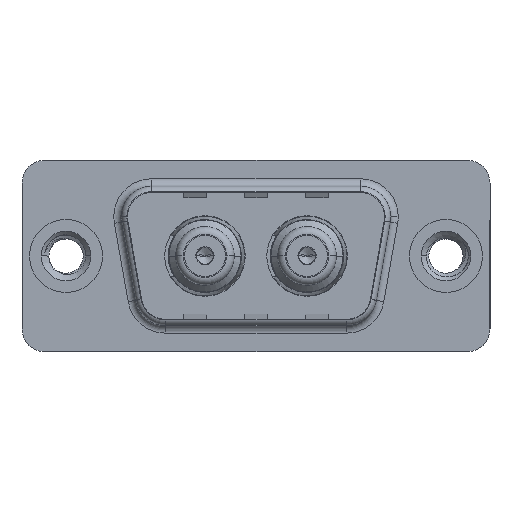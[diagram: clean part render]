
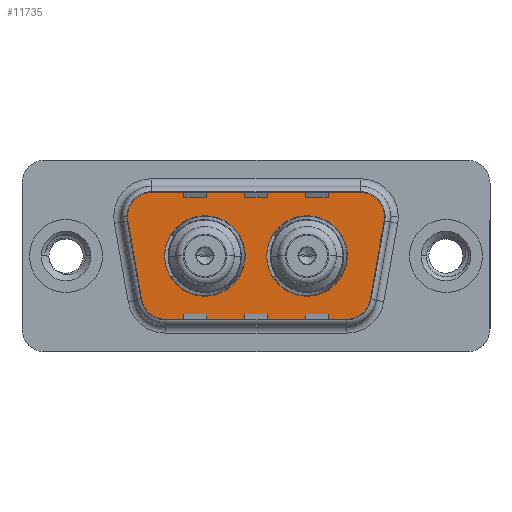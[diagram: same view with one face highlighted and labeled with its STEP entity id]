
A CAD part, top view. The second image highlights one B-rep face of the part: STEP entity #11735.
In plain terms, the highlighted planar face has unit normal (0, 0, 1).
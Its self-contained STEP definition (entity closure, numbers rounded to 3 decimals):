
#1 = CIRCLE ( 'NONE', #564, 2.65 ) ;
#114 = EDGE_CURVE ( 'NONE', #13973, #14673, #2329, .T. ) ;
#326 = VECTOR ( 'NONE', #3303, 1000. ) ;
#469 = DIRECTION ( 'NONE',  ( 0., 0., 1. ) ) ;
#486 = CARTESIAN_POINT ( 'NONE',  ( 19.564, 2.9, 0. ) ) ;
#564 = AXIS2_PLACEMENT_3D ( 'NONE', #6329, #6258, #6147 ) ;
#580 = FACE_BOUND ( 'NONE', #16173, .T. ) ;
#655 = DIRECTION ( 'NONE',  ( -1., 0., 0. ) ) ;
#695 = ORIENTED_EDGE ( 'NONE', *, *, #6274, .T. ) ;
#864 = CARTESIAN_POINT ( 'NONE',  ( 19.564, 2.9, 0. ) ) ;
#968 = CIRCLE ( 'NONE', #18307, 2. ) ;
#1324 = DIRECTION ( 'NONE',  ( 0., 0., 1. ) ) ;
#1358 = EDGE_CURVE ( 'NONE', #16031, #7079, #12045, .T. ) ;
#1480 = VERTEX_POINT ( 'NONE', #13743 ) ;
#1599 = ORIENTED_EDGE ( 'NONE', *, *, #8233, .F. ) ;
#1756 = CIRCLE ( 'NONE', #15174, 2. ) ;
#2310 = DIRECTION ( 'NONE',  ( -1., 0., 0. ) ) ;
#2329 = CIRCLE ( 'NONE', #5282, 2.65 ) ;
#2404 = CIRCLE ( 'NONE', #17236, 2.65 ) ;
#2619 = VERTEX_POINT ( 'NONE', #16301 ) ;
#2859 = CARTESIAN_POINT ( 'NONE',  ( 18.541, -2.9, 0. ) ) ;
#2981 = CARTESIAN_POINT ( 'NONE',  ( 5.436, 2.9, 0. ) ) ;
#3101 = CIRCLE ( 'NONE', #17448, 2. ) ;
#3128 = VECTOR ( 'NONE', #15255, 1000. ) ;
#3303 = DIRECTION ( 'NONE',  ( 0.174, -0.985, 0. ) ) ;
#3501 = FACE_BOUND ( 'NONE', #13004, .T. ) ;
#3754 = CARTESIAN_POINT ( 'NONE',  ( 5.436, 4.9, 0. ) ) ;
#4258 = DIRECTION ( 'NONE',  ( 1., 0., 0. ) ) ;
#4263 = EDGE_CURVE ( 'NONE', #13806, #17705, #1, .T. ) ;
#4389 = DIRECTION ( 'NONE',  ( 1., 0., 0. ) ) ;
#4454 = EDGE_CURVE ( 'NONE', #15812, #12667, #9995, .T. ) ;
#4488 = CIRCLE ( 'NONE', #15249, 2. ) ;
#4517 = CARTESIAN_POINT ( 'NONE',  ( 3.466, 2.553, 0. ) ) ;
#5018 = EDGE_CURVE ( 'NONE', #12593, #1480, #17698, .T. ) ;
#5043 = EDGE_CURVE ( 'NONE', #16084, #15812, #10149, .T. ) ;
#5282 = AXIS2_PLACEMENT_3D ( 'NONE', #17129, #10798, #13924 ) ;
#5322 = VECTOR ( 'NONE', #15487, 1000. ) ;
#5355 = CARTESIAN_POINT ( 'NONE',  ( 9.14, 0., 0. ) ) ;
#5369 = DIRECTION ( 'NONE',  ( -1., 0., 0. ) ) ;
#5607 = CARTESIAN_POINT ( 'NONE',  ( 21.534, 2.553, 0. ) ) ;
#5785 = VERTEX_POINT ( 'NONE', #6048 ) ;
#6048 = CARTESIAN_POINT ( 'NONE',  ( 21.534, 2.553, 0. ) ) ;
#6147 = DIRECTION ( 'NONE',  ( 1., 0., 0. ) ) ;
#6219 = ORIENTED_EDGE ( 'NONE', *, *, #18273, .T. ) ;
#6258 = DIRECTION ( 'NONE',  ( 0., 0., 1. ) ) ;
#6274 = EDGE_CURVE ( 'NONE', #1480, #2619, #3101, .T. ) ;
#6329 = CARTESIAN_POINT ( 'NONE',  ( 9.14, 0., 0. ) ) ;
#6382 = CARTESIAN_POINT ( 'NONE',  ( 6.459, -4.9, 0. ) ) ;
#6734 = DIRECTION ( 'NONE',  ( 1., 0., 0. ) ) ;
#7079 = VERTEX_POINT ( 'NONE', #10060 ) ;
#7116 = ORIENTED_EDGE ( 'NONE', *, *, #4454, .T. ) ;
#7161 = CARTESIAN_POINT ( 'NONE',  ( 18.51, 0., 0. ) ) ;
#7391 = CARTESIAN_POINT ( 'NONE',  ( 3.466, 2.553, 0. ) ) ;
#7783 = ORIENTED_EDGE ( 'NONE', *, *, #5043, .T. ) ;
#7798 = ORIENTED_EDGE ( 'NONE', *, *, #9588, .T. ) ;
#8108 = CARTESIAN_POINT ( 'NONE',  ( 6.459, -2.9, 0. ) ) ;
#8119 = CARTESIAN_POINT ( 'NONE',  ( 5.436, 4.9, 0. ) ) ;
#8124 = CARTESIAN_POINT ( 'NONE',  ( 15.86, 0., 0. ) ) ;
#8233 = EDGE_CURVE ( 'NONE', #14673, #13973, #2404, .T. ) ;
#8450 = ORIENTED_EDGE ( 'NONE', *, *, #16518, .T. ) ;
#8786 = CIRCLE ( 'NONE', #17103, 2.65 ) ;
#9030 = LINE ( 'NONE', #5607, #5322 ) ;
#9506 = DIRECTION ( 'NONE',  ( -1., 0., 0. ) ) ;
#9523 = DIRECTION ( 'NONE',  ( 1., 0., 0. ) ) ;
#9588 = EDGE_CURVE ( 'NONE', #7079, #12593, #1756, .T. ) ;
#9617 = EDGE_CURVE ( 'NONE', #17705, #13806, #8786, .T. ) ;
#9743 = CARTESIAN_POINT ( 'NONE',  ( 18.541, -2.9, 0. ) ) ;
#9995 = LINE ( 'NONE', #8119, #12392 ) ;
#10060 = CARTESIAN_POINT ( 'NONE',  ( 4.489, -3.247, 0. ) ) ;
#10149 = CIRCLE ( 'NONE', #12141, 2. ) ;
#10189 = ORIENTED_EDGE ( 'NONE', *, *, #4263, .F. ) ;
#10729 = DIRECTION ( 'NONE',  ( 0., 0., 1. ) ) ;
#10798 = DIRECTION ( 'NONE',  ( 0., 0., 1. ) ) ;
#11169 = DIRECTION ( 'NONE',  ( 1., 0., 0. ) ) ;
#11325 = CARTESIAN_POINT ( 'NONE',  ( 13.21, 0., 0. ) ) ;
#11396 = CARTESIAN_POINT ( 'NONE',  ( 11.79, 0., 0. ) ) ;
#11735 = ADVANCED_FACE ( 'NONE', ( #580, #3501, #18072 ), #13940, .T. ) ;
#12045 = LINE ( 'NONE', #7391, #326 ) ;
#12141 = AXIS2_PLACEMENT_3D ( 'NONE', #486, #469, #655 ) ;
#12392 = VECTOR ( 'NONE', #5369, 1000. ) ;
#12593 = VERTEX_POINT ( 'NONE', #6382 ) ;
#12641 = DIRECTION ( 'NONE',  ( 0., 0., 1. ) ) ;
#12667 = VERTEX_POINT ( 'NONE', #3754 ) ;
#12784 = DIRECTION ( 'NONE',  ( 0., 0., 1. ) ) ;
#12850 = ORIENTED_EDGE ( 'NONE', *, *, #5018, .T. ) ;
#13004 = EDGE_LOOP ( 'NONE', ( #14146, #10189 ) ) ;
#13518 = ORIENTED_EDGE ( 'NONE', *, *, #1358, .T. ) ;
#13743 = CARTESIAN_POINT ( 'NONE',  ( 18.541, -4.9, 0. ) ) ;
#13806 = VERTEX_POINT ( 'NONE', #16797 ) ;
#13924 = DIRECTION ( 'NONE',  ( 1., 0., 0. ) ) ;
#13940 = PLANE ( 'NONE',  #18388 ) ;
#13973 = VERTEX_POINT ( 'NONE', #7161 ) ;
#14146 = ORIENTED_EDGE ( 'NONE', *, *, #9617, .F. ) ;
#14673 = VERTEX_POINT ( 'NONE', #11325 ) ;
#14932 = EDGE_CURVE ( 'NONE', #5785, #16084, #968, .T. ) ;
#15106 = EDGE_LOOP ( 'NONE', ( #695, #6219, #17322, #7783, #7116, #8450, #13518, #7798, #12850 ) ) ;
#15174 = AXIS2_PLACEMENT_3D ( 'NONE', #8108, #18001, #9506 ) ;
#15223 = DIRECTION ( 'NONE',  ( 0., 0., 1. ) ) ;
#15249 = AXIS2_PLACEMENT_3D ( 'NONE', #2981, #12784, #4389 ) ;
#15255 = DIRECTION ( 'NONE',  ( 1., 0., 0. ) ) ;
#15487 = DIRECTION ( 'NONE',  ( 0.174, 0.985, 0. ) ) ;
#15812 = VERTEX_POINT ( 'NONE', #16418 ) ;
#16031 = VERTEX_POINT ( 'NONE', #4517 ) ;
#16084 = VERTEX_POINT ( 'NONE', #17309 ) ;
#16173 = EDGE_LOOP ( 'NONE', ( #16397, #1599 ) ) ;
#16301 = CARTESIAN_POINT ( 'NONE',  ( 20.511, -3.247, 0. ) ) ;
#16342 = CARTESIAN_POINT ( 'NONE',  ( 6.459, -4.9, 0. ) ) ;
#16397 = ORIENTED_EDGE ( 'NONE', *, *, #114, .F. ) ;
#16418 = CARTESIAN_POINT ( 'NONE',  ( 19.564, 4.9, 0. ) ) ;
#16518 = EDGE_CURVE ( 'NONE', #12667, #16031, #4488, .T. ) ;
#16797 = CARTESIAN_POINT ( 'NONE',  ( 6.49, 0., 0. ) ) ;
#17103 = AXIS2_PLACEMENT_3D ( 'NONE', #5355, #15223, #6734 ) ;
#17129 = CARTESIAN_POINT ( 'NONE',  ( 15.86, 0., 0. ) ) ;
#17236 = AXIS2_PLACEMENT_3D ( 'NONE', #8124, #18021, #9523 ) ;
#17309 = CARTESIAN_POINT ( 'NONE',  ( 21.564, 2.9, 0. ) ) ;
#17322 = ORIENTED_EDGE ( 'NONE', *, *, #14932, .T. ) ;
#17448 = AXIS2_PLACEMENT_3D ( 'NONE', #2859, #12641, #4258 ) ;
#17698 = LINE ( 'NONE', #16342, #3128 ) ;
#17705 = VERTEX_POINT ( 'NONE', #11396 ) ;
#18001 = DIRECTION ( 'NONE',  ( 0., 0., 1. ) ) ;
#18021 = DIRECTION ( 'NONE',  ( 0., 0., 1. ) ) ;
#18072 = FACE_OUTER_BOUND ( 'NONE', #15106, .T. ) ;
#18273 = EDGE_CURVE ( 'NONE', #2619, #5785, #9030, .T. ) ;
#18307 = AXIS2_PLACEMENT_3D ( 'NONE', #864, #10729, #2310 ) ;
#18388 = AXIS2_PLACEMENT_3D ( 'NONE', #9743, #1324, #11169 ) ;
